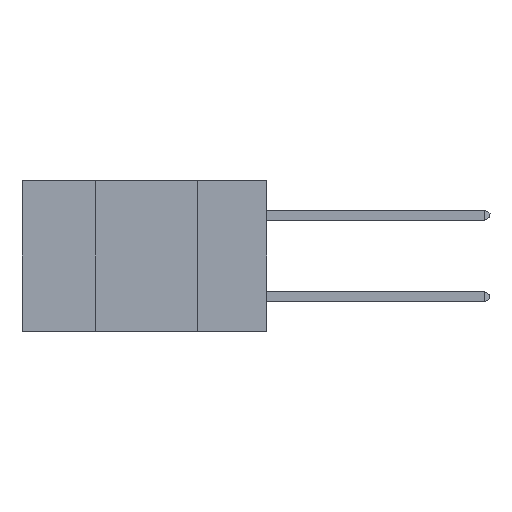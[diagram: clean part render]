
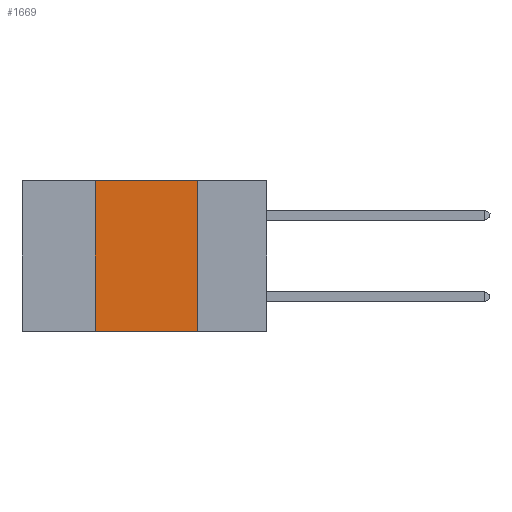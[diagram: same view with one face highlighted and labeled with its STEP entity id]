
A CAD part, left-side view. The second image highlights one B-rep face of the part: STEP entity #1669.
In plain terms, the highlighted planar face has unit normal (-1, 0, 0).
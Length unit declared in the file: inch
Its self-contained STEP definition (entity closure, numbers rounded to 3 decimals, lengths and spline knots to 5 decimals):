
#116 = DIRECTION ( 'NONE',  ( 0., -1., 0. ) ) ;
#122 = CARTESIAN_POINT ( 'NONE',  ( 0., 0.6, 0. ) ) ;
#155 = CARTESIAN_POINT ( 'NONE',  ( 0., 0.17, 0. ) ) ;
#782 = VERTEX_POINT ( 'NONE', #5188 ) ;
#1316 = DIRECTION ( 'NONE',  ( 0., -1., 0. ) ) ;
#1338 = DIRECTION ( 'NONE',  ( 0., 0., -1. ) ) ;
#1402 = FACE_OUTER_BOUND ( 'NONE', #5237, .T. ) ;
#1669 = ADVANCED_FACE ( 'NONE', ( #1402 ), #10226, .F. ) ;
#1819 = ORIENTED_EDGE ( 'NONE', *, *, #8881, .F. ) ;
#3922 = DIRECTION ( 'NONE',  ( 1., 0., 0. ) ) ;
#3996 = VECTOR ( 'NONE', #1338, 39.37008 ) ;
#4069 = LINE ( 'NONE', #6955, #6458 ) ;
#4297 = EDGE_CURVE ( 'NONE', #782, #5214, #6135, .T. ) ;
#4500 = DIRECTION ( 'NONE',  ( 0., 0., 1. ) ) ;
#5105 = CARTESIAN_POINT ( 'NONE',  ( 0., 0.42, 0. ) ) ;
#5188 = CARTESIAN_POINT ( 'NONE',  ( 0., 0.17, 0. ) ) ;
#5214 = VERTEX_POINT ( 'NONE', #7200 ) ;
#5237 = EDGE_LOOP ( 'NONE', ( #8464, #1819, #11316, #9105 ) ) ;
#5896 = EDGE_CURVE ( 'NONE', #8283, #6350, #7557, .T. ) ;
#6115 = AXIS2_PLACEMENT_3D ( 'NONE', #10088, #3922, #10862 ) ;
#6135 = LINE ( 'NONE', #155, #3996 ) ;
#6350 = VERTEX_POINT ( 'NONE', #5105 ) ;
#6458 = VECTOR ( 'NONE', #116, 39.37008 ) ;
#6610 = LINE ( 'NONE', #122, #8568 ) ;
#6955 = CARTESIAN_POINT ( 'NONE',  ( 0., 0.6, -0.37 ) ) ;
#7115 = CARTESIAN_POINT ( 'NONE',  ( 0., 0.42, 0. ) ) ;
#7200 = CARTESIAN_POINT ( 'NONE',  ( 0., 0.17, -0.37 ) ) ;
#7557 = LINE ( 'NONE', #7115, #11559 ) ;
#8283 = VERTEX_POINT ( 'NONE', #10309 ) ;
#8464 = ORIENTED_EDGE ( 'NONE', *, *, #4297, .F. ) ;
#8568 = VECTOR ( 'NONE', #1316, 39.37008 ) ;
#8881 = EDGE_CURVE ( 'NONE', #6350, #782, #6610, .T. ) ;
#9105 = ORIENTED_EDGE ( 'NONE', *, *, #10905, .T. ) ;
#10088 = CARTESIAN_POINT ( 'NONE',  ( 0., 0.6, 0. ) ) ;
#10226 = PLANE ( 'NONE',  #6115 ) ;
#10309 = CARTESIAN_POINT ( 'NONE',  ( 0., 0.42, -0.37 ) ) ;
#10862 = DIRECTION ( 'NONE',  ( 0., 0., -1. ) ) ;
#10905 = EDGE_CURVE ( 'NONE', #8283, #5214, #4069, .T. ) ;
#11316 = ORIENTED_EDGE ( 'NONE', *, *, #5896, .F. ) ;
#11559 = VECTOR ( 'NONE', #4500, 39.37008 ) ;
